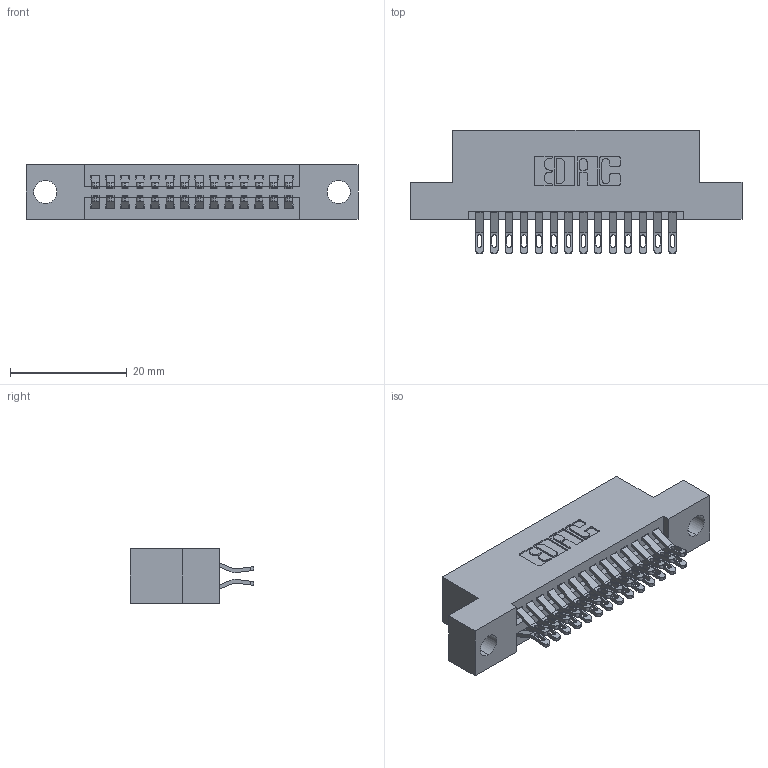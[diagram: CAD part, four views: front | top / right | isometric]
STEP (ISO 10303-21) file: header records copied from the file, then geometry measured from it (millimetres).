
FILE_DESCRIPTION (( 'STEP AP203' ), '1' );
FILE_NAME ('345-028-555-204.STEP', '2021-05-19T23:08:08', ( '' ), ( '' ), 'SwSTEP 2.0', 'SolidWorks 2020', '' );
FILE_SCHEMA (( 'CONFIG_CONTROL_DESIGN' ));
Length unit declared in the file: inch
Products named in the file (3): 345-028-555-204; 345 Part_Flush Mounting Lugs - 0.156 Dia-TI; 345-292-001_555 Tail
Assembly tree (29 placements, depth 2):
  345-028-555-204
    345 Part_Flush Mounting Lugs - 0.156 Dia-TI
    345-292-001_555 Tail  x28
Bounding box: 56.77 x 21.13 x 9.4 mm (x, y, z)
Volume: 5230 mm3; surface area: 7322.5 mm2
Topology: 29 solids, 29 shells, 1708 faces, 5333 edges, 3554 vertices
Faces by surface type: plane 962, cylinder 746
Entity records: 15499 total; most frequent: CARTESIAN_POINT 2664, ORIENTED_EDGE 2566, DIRECTION 2351, EDGE_CURVE 1283, LINE 1075, VECTOR 1075, VERTEX_POINT 854, AXIS2_PLACEMENT_3D 638
